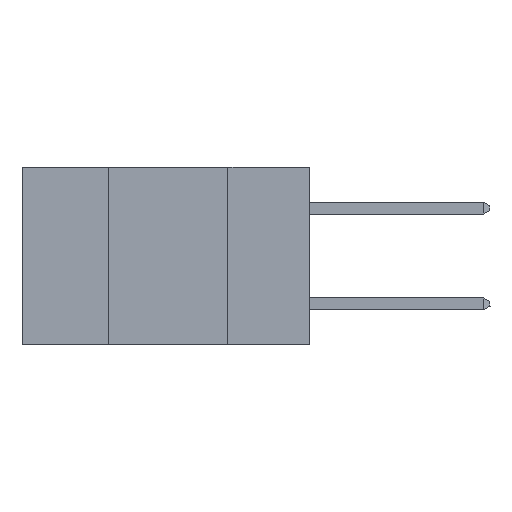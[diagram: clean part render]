
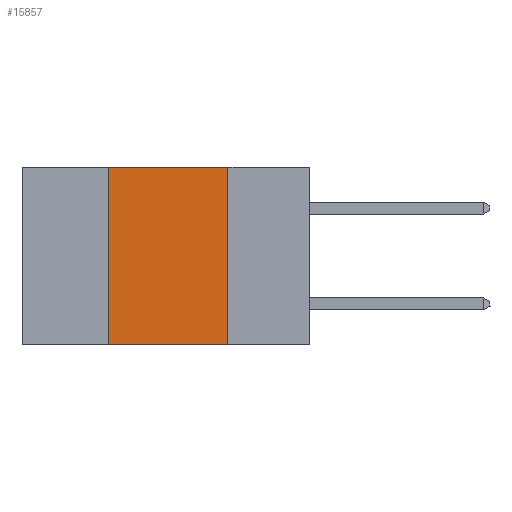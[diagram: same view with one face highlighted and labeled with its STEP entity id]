
A CAD part, left-side view. The second image highlights one B-rep face of the part: STEP entity #15857.
In plain terms, the highlighted planar face has unit normal (-1, 0, 0).
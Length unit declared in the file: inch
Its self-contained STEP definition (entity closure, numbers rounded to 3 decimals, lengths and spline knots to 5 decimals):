
#922 = AXIS2_PLACEMENT_3D ( 'NONE', #18435, #15026, #8198 ) ;
#1169 = ORIENTED_EDGE ( 'NONE', *, *, #9484, .F. ) ;
#1287 = DIRECTION ( 'NONE',  ( 0., -1., 0. ) ) ;
#1813 = CARTESIAN_POINT ( 'NONE',  ( 0., 0.42, 0. ) ) ;
#2147 = DIRECTION ( 'NONE',  ( 0., 0., 1. ) ) ;
#2710 = DIRECTION ( 'NONE',  ( 0., -1., 0. ) ) ;
#2822 = CARTESIAN_POINT ( 'NONE',  ( 0., 0.6, -0.37 ) ) ;
#3298 = DIRECTION ( 'NONE',  ( 0., 0., -1. ) ) ;
#3325 = EDGE_CURVE ( 'NONE', #21297, #18678, #16832, .T. ) ;
#3644 = EDGE_CURVE ( 'NONE', #8119, #18678, #9984, .T. ) ;
#3759 = LINE ( 'NONE', #1813, #17846 ) ;
#4689 = EDGE_CURVE ( 'NONE', #8119, #6819, #3759, .T. ) ;
#5870 = VECTOR ( 'NONE', #2710, 39.37008 ) ;
#6142 = ORIENTED_EDGE ( 'NONE', *, *, #3644, .T. ) ;
#6819 = VERTEX_POINT ( 'NONE', #14690 ) ;
#7670 = CARTESIAN_POINT ( 'NONE',  ( 0., 0.17, -0.37 ) ) ;
#8119 = VERTEX_POINT ( 'NONE', #9588 ) ;
#8183 = CARTESIAN_POINT ( 'NONE',  ( 0., 0.17, 0. ) ) ;
#8198 = DIRECTION ( 'NONE',  ( 0., 0., -1. ) ) ;
#9484 = EDGE_CURVE ( 'NONE', #6819, #21297, #14956, .T. ) ;
#9582 = ORIENTED_EDGE ( 'NONE', *, *, #3325, .F. ) ;
#9588 = CARTESIAN_POINT ( 'NONE',  ( 0., 0.42, -0.37 ) ) ;
#9984 = LINE ( 'NONE', #2822, #5870 ) ;
#10686 = ORIENTED_EDGE ( 'NONE', *, *, #4689, .F. ) ;
#13099 = FACE_OUTER_BOUND ( 'NONE', #14643, .T. ) ;
#13480 = CARTESIAN_POINT ( 'NONE',  ( 0., 0.6, 0. ) ) ;
#13762 = VECTOR ( 'NONE', #1287, 39.37008 ) ;
#14643 = EDGE_LOOP ( 'NONE', ( #9582, #1169, #10686, #6142 ) ) ;
#14690 = CARTESIAN_POINT ( 'NONE',  ( 0., 0.42, 0. ) ) ;
#14956 = LINE ( 'NONE', #13480, #13762 ) ;
#15026 = DIRECTION ( 'NONE',  ( 1., 0., 0. ) ) ;
#15857 = ADVANCED_FACE ( 'NONE', ( #13099 ), #20141, .F. ) ;
#16832 = LINE ( 'NONE', #22308, #21854 ) ;
#17846 = VECTOR ( 'NONE', #2147, 39.37008 ) ;
#18435 = CARTESIAN_POINT ( 'NONE',  ( 0., 0.6, 0. ) ) ;
#18678 = VERTEX_POINT ( 'NONE', #7670 ) ;
#20141 = PLANE ( 'NONE',  #922 ) ;
#21297 = VERTEX_POINT ( 'NONE', #8183 ) ;
#21854 = VECTOR ( 'NONE', #3298, 39.37008 ) ;
#22308 = CARTESIAN_POINT ( 'NONE',  ( 0., 0.17, 0. ) ) ;
